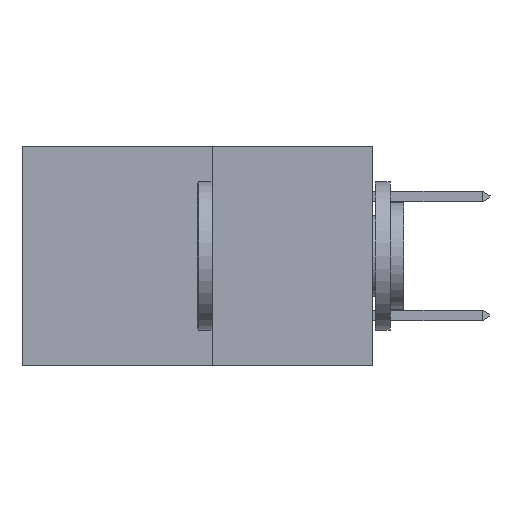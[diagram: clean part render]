
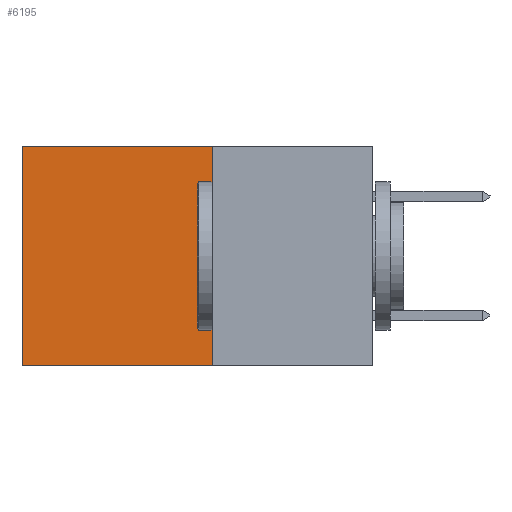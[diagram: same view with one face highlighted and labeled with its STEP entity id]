
A CAD part, left-side view. The second image highlights one B-rep face of the part: STEP entity #6195.
In plain terms, the highlighted planar face has unit normal (-1, 0, 0).
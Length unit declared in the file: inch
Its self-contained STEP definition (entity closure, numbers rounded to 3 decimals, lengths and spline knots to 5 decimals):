
#742 = EDGE_CURVE ( 'NONE', #5721, #9258, #7215, .T. ) ;
#776 = DIRECTION ( 'NONE',  ( 0., 0., -1. ) ) ;
#1475 = CARTESIAN_POINT ( 'NONE',  ( 0.277, 0.27, -0.37 ) ) ;
#1529 = LINE ( 'NONE', #9285, #2204 ) ;
#2204 = VECTOR ( 'NONE', #3175, 39.37008 ) ;
#3092 = EDGE_CURVE ( 'NONE', #11540, #8133, #4782, .T. ) ;
#3175 = DIRECTION ( 'NONE',  ( 0., 1., 0. ) ) ;
#3798 = CARTESIAN_POINT ( 'NONE',  ( 0.277, 0.59, -0.37 ) ) ;
#4150 = CARTESIAN_POINT ( 'NONE',  ( 0.277, 0.27, 0. ) ) ;
#4782 = LINE ( 'NONE', #8156, #9847 ) ;
#5527 = FACE_OUTER_BOUND ( 'NONE', #9529, .T. ) ;
#5559 = DIRECTION ( 'NONE',  ( 0., 0., -1. ) ) ;
#5568 = AXIS2_PLACEMENT_3D ( 'NONE', #10029, #7030, #776 ) ;
#5721 = VERTEX_POINT ( 'NONE', #4150 ) ;
#5818 = DIRECTION ( 'NONE',  ( 0., 1., 0. ) ) ;
#6195 = ADVANCED_FACE ( 'NONE', ( #5527 ), #12079, .F. ) ;
#6598 = CARTESIAN_POINT ( 'NONE',  ( 0.277, 0.27, -0.37 ) ) ;
#7030 = DIRECTION ( 'NONE',  ( 1., 0., 0. ) ) ;
#7215 = LINE ( 'NONE', #1475, #10563 ) ;
#8133 = VERTEX_POINT ( 'NONE', #3798 ) ;
#8156 = CARTESIAN_POINT ( 'NONE',  ( 0.277, 0.59, -0.37 ) ) ;
#9258 = VERTEX_POINT ( 'NONE', #6598 ) ;
#9261 = VECTOR ( 'NONE', #5818, 39.37008 ) ;
#9285 = CARTESIAN_POINT ( 'NONE',  ( 0.277, 0.27, 0. ) ) ;
#9457 = EDGE_CURVE ( 'NONE', #9258, #8133, #9931, .T. ) ;
#9526 = ORIENTED_EDGE ( 'NONE', *, *, #3092, .T. ) ;
#9529 = EDGE_LOOP ( 'NONE', ( #9526, #9631, #9777, #9731 ) ) ;
#9631 = ORIENTED_EDGE ( 'NONE', *, *, #9457, .F. ) ;
#9703 = EDGE_CURVE ( 'NONE', #5721, #11540, #1529, .T. ) ;
#9731 = ORIENTED_EDGE ( 'NONE', *, *, #9703, .T. ) ;
#9777 = ORIENTED_EDGE ( 'NONE', *, *, #742, .F. ) ;
#9801 = CARTESIAN_POINT ( 'NONE',  ( 0.277, 0.27, -0.37 ) ) ;
#9847 = VECTOR ( 'NONE', #5559, 39.37008 ) ;
#9931 = LINE ( 'NONE', #9801, #9261 ) ;
#10029 = CARTESIAN_POINT ( 'NONE',  ( 0.277, 0.27, -0.37 ) ) ;
#10563 = VECTOR ( 'NONE', #10685, 39.37008 ) ;
#10685 = DIRECTION ( 'NONE',  ( 0., 0., -1. ) ) ;
#11540 = VERTEX_POINT ( 'NONE', #12317 ) ;
#12079 = PLANE ( 'NONE',  #5568 ) ;
#12317 = CARTESIAN_POINT ( 'NONE',  ( 0.277, 0.59, 0. ) ) ;
